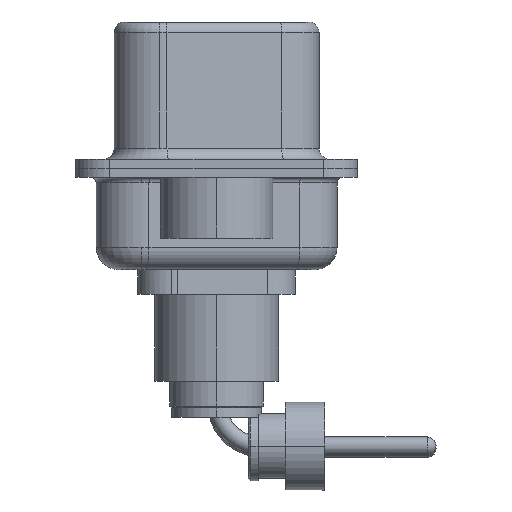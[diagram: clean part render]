
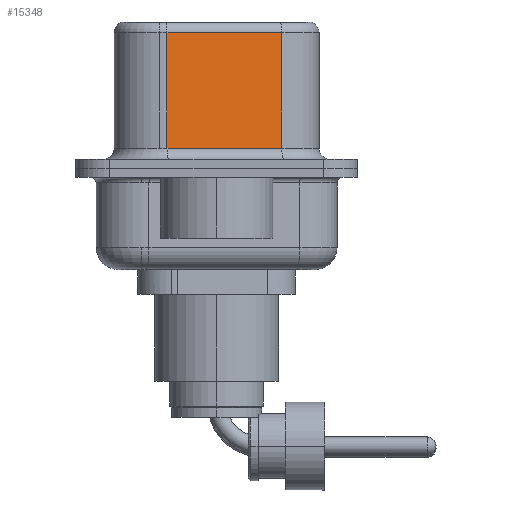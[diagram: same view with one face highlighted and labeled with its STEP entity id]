
A CAD part, left-side view. The second image highlights one B-rep face of the part: STEP entity #15348.
In plain terms, the highlighted planar face has unit normal (-0.985, -0.174, 0).
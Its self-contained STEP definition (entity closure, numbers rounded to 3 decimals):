
#862 = CARTESIAN_POINT ( 'NONE',  ( 4.555, -2.897, 6.52 ) ) ;
#1445 = EDGE_CURVE ( 'NONE', #17375, #2104, #18917, .T. ) ;
#1847 = EDGE_CURVE ( 'NONE', #19576, #15040, #18002, .T. ) ;
#2096 = DIRECTION ( 'NONE',  ( -0.174, 0.985, 0. ) ) ;
#2104 = VERTEX_POINT ( 'NONE', #14462 ) ;
#2955 = VECTOR ( 'NONE', #2096, 1000. ) ;
#3509 = CARTESIAN_POINT ( 'NONE',  ( 4.555, -2.897, 6.02 ) ) ;
#3878 = CARTESIAN_POINT ( 'NONE',  ( 4.555, -2.897, 6.52 ) ) ;
#4316 = CARTESIAN_POINT ( 'NONE',  ( 4.555, -2.897, 0.9 ) ) ;
#5412 = VECTOR ( 'NONE', #8697, 1000. ) ;
#5872 = CARTESIAN_POINT ( 'NONE',  ( 3.655, 2.203, 6.52 ) ) ;
#6857 = ORIENTED_EDGE ( 'NONE', *, *, #16527, .T. ) ;
#7369 = LINE ( 'NONE', #5872, #11460 ) ;
#7483 = VECTOR ( 'NONE', #13553, 1000. ) ;
#8297 = FACE_OUTER_BOUND ( 'NONE', #10673, .T. ) ;
#8697 = DIRECTION ( 'NONE',  ( 0., 0., -1. ) ) ;
#10200 = DIRECTION ( 'NONE',  ( -0.174, 0.985, 0. ) ) ;
#10673 = EDGE_LOOP ( 'NONE', ( #15435, #11775, #6857, #10946 ) ) ;
#10946 = ORIENTED_EDGE ( 'NONE', *, *, #1847, .T. ) ;
#11460 = VECTOR ( 'NONE', #18144, 1000. ) ;
#11775 = ORIENTED_EDGE ( 'NONE', *, *, #1445, .T. ) ;
#13553 = DIRECTION ( 'NONE',  ( 0.174, -0.985, 0. ) ) ;
#13907 = CARTESIAN_POINT ( 'NONE',  ( 3.655, 2.203, 0.9 ) ) ;
#14448 = PLANE ( 'NONE',  #18825 ) ;
#14462 = CARTESIAN_POINT ( 'NONE',  ( 3.655, 2.203, 6.02 ) ) ;
#15040 = VERTEX_POINT ( 'NONE', #17483 ) ;
#15079 = CARTESIAN_POINT ( 'NONE',  ( 4.555, -2.897, 6.02 ) ) ;
#15348 = ADVANCED_FACE ( 'NONE', ( #8297 ), #14448, .F. ) ;
#15435 = ORIENTED_EDGE ( 'NONE', *, *, #17709, .F. ) ;
#16527 = EDGE_CURVE ( 'NONE', #2104, #19576, #7369, .T. ) ;
#17375 = VERTEX_POINT ( 'NONE', #15079 ) ;
#17483 = CARTESIAN_POINT ( 'NONE',  ( 4.555, -2.897, 0.9 ) ) ;
#17709 = EDGE_CURVE ( 'NONE', #17375, #15040, #19393, .T. ) ;
#17771 = DIRECTION ( 'NONE',  ( 0.985, 0.174, 0. ) ) ;
#18002 = LINE ( 'NONE', #4316, #7483 ) ;
#18144 = DIRECTION ( 'NONE',  ( 0., 0., -1. ) ) ;
#18825 = AXIS2_PLACEMENT_3D ( 'NONE', #3878, #17771, #10200 ) ;
#18917 = LINE ( 'NONE', #3509, #2955 ) ;
#19393 = LINE ( 'NONE', #862, #5412 ) ;
#19576 = VERTEX_POINT ( 'NONE', #13907 ) ;
